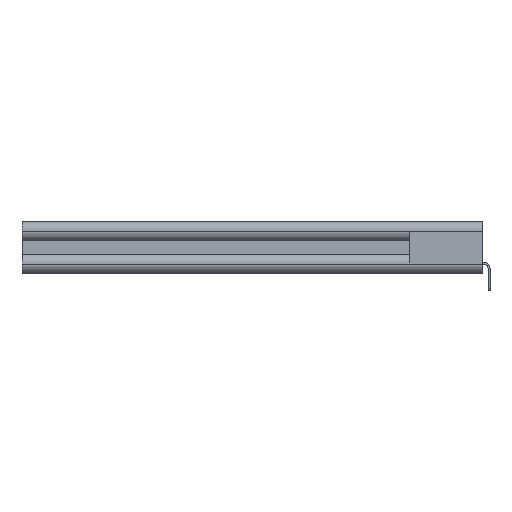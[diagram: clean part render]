
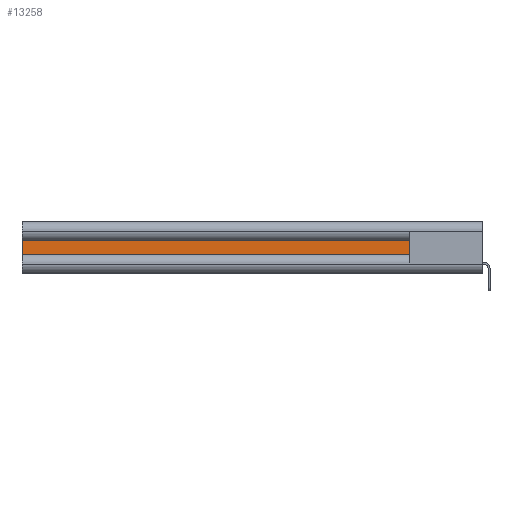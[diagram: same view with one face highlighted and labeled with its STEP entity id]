
A CAD part, left-side view. The second image highlights one B-rep face of the part: STEP entity #13258.
In plain terms, the highlighted planar face has unit normal (-1, 0, 0).
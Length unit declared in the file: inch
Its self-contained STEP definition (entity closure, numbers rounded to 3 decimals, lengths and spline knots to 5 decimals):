
#373 = DIRECTION ( 'NONE',  ( 0., 1., 0. ) ) ;
#1085 = CARTESIAN_POINT ( 'NONE',  ( 0.044, 0.37012, 0.0465 ) ) ;
#1654 = VECTOR ( 'NONE', #1810, 39.37008 ) ;
#1810 = DIRECTION ( 'NONE',  ( 0., 0., -1. ) ) ;
#1841 = AXIS2_PLACEMENT_3D ( 'NONE', #6544, #19168, #8421 ) ;
#1850 = CARTESIAN_POINT ( 'NONE',  ( 0.044, 0.473, -0.0465 ) ) ;
#3553 = ORIENTED_EDGE ( 'NONE', *, *, #18865, .T. ) ;
#4614 = LINE ( 'NONE', #5221, #8361 ) ;
#5221 = CARTESIAN_POINT ( 'NONE',  ( 0.044, 0.473, -0.0465 ) ) ;
#5232 = EDGE_CURVE ( 'NONE', #16001, #11825, #13808, .T. ) ;
#6468 = PLANE ( 'NONE',  #1841 ) ;
#6544 = CARTESIAN_POINT ( 'NONE',  ( 0.044, 0.37012, -0.0465 ) ) ;
#6609 = LINE ( 'NONE', #9199, #1654 ) ;
#8361 = VECTOR ( 'NONE', #19636, 39.37008 ) ;
#8421 = DIRECTION ( 'NONE',  ( 0., 0., -1. ) ) ;
#9199 = CARTESIAN_POINT ( 'NONE',  ( 0.044, 3., -0.0465 ) ) ;
#9602 = CARTESIAN_POINT ( 'NONE',  ( 0.044, 0.473, 0.0465 ) ) ;
#9829 = CARTESIAN_POINT ( 'NONE',  ( 0.044, 3., 0.0465 ) ) ;
#10221 = DIRECTION ( 'NONE',  ( 0., 1., 0. ) ) ;
#10298 = ORIENTED_EDGE ( 'NONE', *, *, #22409, .F. ) ;
#11825 = VERTEX_POINT ( 'NONE', #12820 ) ;
#11999 = VERTEX_POINT ( 'NONE', #9829 ) ;
#12820 = CARTESIAN_POINT ( 'NONE',  ( 0.044, 3., -0.0465 ) ) ;
#13258 = ADVANCED_FACE ( 'NONE', ( #17380 ), #6468, .F. ) ;
#13297 = ORIENTED_EDGE ( 'NONE', *, *, #5232, .F. ) ;
#13808 = LINE ( 'NONE', #22062, #22635 ) ;
#15829 = ORIENTED_EDGE ( 'NONE', *, *, #21874, .T. ) ;
#16001 = VERTEX_POINT ( 'NONE', #1850 ) ;
#17257 = VECTOR ( 'NONE', #10221, 39.37008 ) ;
#17380 = FACE_OUTER_BOUND ( 'NONE', #19137, .T. ) ;
#18865 = EDGE_CURVE ( 'NONE', #20586, #11999, #21335, .T. ) ;
#19137 = EDGE_LOOP ( 'NONE', ( #3553, #15829, #13297, #10298 ) ) ;
#19168 = DIRECTION ( 'NONE',  ( 1., 0., 0. ) ) ;
#19636 = DIRECTION ( 'NONE',  ( 0., 0., -1. ) ) ;
#20586 = VERTEX_POINT ( 'NONE', #9602 ) ;
#21335 = LINE ( 'NONE', #1085, #17257 ) ;
#21874 = EDGE_CURVE ( 'NONE', #11999, #11825, #6609, .T. ) ;
#22062 = CARTESIAN_POINT ( 'NONE',  ( 0.044, 0.37012, -0.0465 ) ) ;
#22409 = EDGE_CURVE ( 'NONE', #20586, #16001, #4614, .T. ) ;
#22635 = VECTOR ( 'NONE', #373, 39.37008 ) ;
